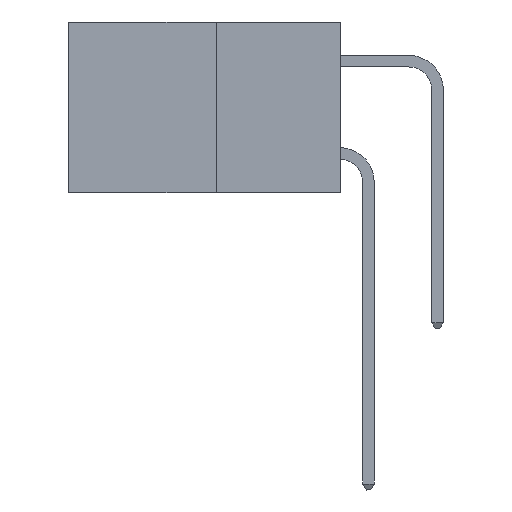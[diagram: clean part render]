
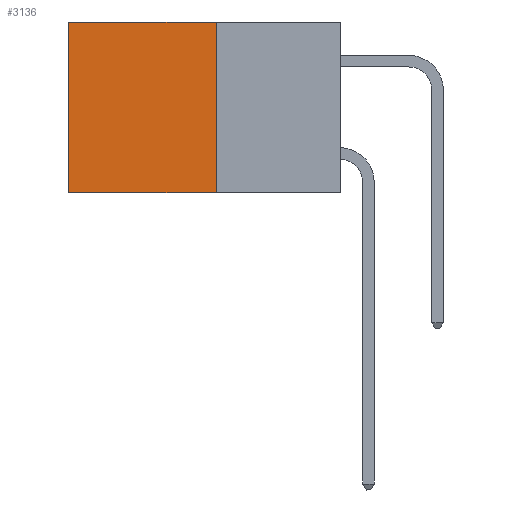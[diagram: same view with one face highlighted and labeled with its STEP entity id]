
A CAD part, left-side view. The second image highlights one B-rep face of the part: STEP entity #3136.
In plain terms, the highlighted planar face has unit normal (-1, 0, 0).
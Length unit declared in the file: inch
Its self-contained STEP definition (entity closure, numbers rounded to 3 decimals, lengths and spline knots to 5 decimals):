
#578 = LINE ( 'NONE', #8632, #11814 ) ;
#2811 = ORIENTED_EDGE ( 'NONE', *, *, #6067, .T. ) ;
#2871 = EDGE_CURVE ( 'NONE', #19294, #12877, #27606, .T. ) ;
#3136 = ADVANCED_FACE ( 'NONE', ( #26526 ), #15058, .F. ) ;
#6067 = EDGE_CURVE ( 'NONE', #19294, #20197, #23130, .T. ) ;
#6079 = CARTESIAN_POINT ( 'NONE',  ( 0.277, 0.59, -0.37 ) ) ;
#8632 = CARTESIAN_POINT ( 'NONE',  ( 0.277, 0.59, -0.37 ) ) ;
#8662 = CARTESIAN_POINT ( 'NONE',  ( 0.277, 0.27, -0.37 ) ) ;
#9228 = ORIENTED_EDGE ( 'NONE', *, *, #24205, .T. ) ;
#10613 = VECTOR ( 'NONE', #25537, 39.37008 ) ;
#10832 = CARTESIAN_POINT ( 'NONE',  ( 0.277, 0.27, 0. ) ) ;
#10877 = DIRECTION ( 'NONE',  ( 0., 0., -1. ) ) ;
#11814 = VECTOR ( 'NONE', #10877, 39.37008 ) ;
#12596 = ORIENTED_EDGE ( 'NONE', *, *, #24712, .F. ) ;
#12877 = VERTEX_POINT ( 'NONE', #8662 ) ;
#14451 = CARTESIAN_POINT ( 'NONE',  ( 0.277, 0.27, 0. ) ) ;
#14726 = DIRECTION ( 'NONE',  ( 0., 0., -1. ) ) ;
#14819 = DIRECTION ( 'NONE',  ( 1., 0., 0. ) ) ;
#15058 = PLANE ( 'NONE',  #26820 ) ;
#15574 = CARTESIAN_POINT ( 'NONE',  ( 0.277, 0.27, -0.37 ) ) ;
#16291 = VECTOR ( 'NONE', #23583, 39.37008 ) ;
#16881 = ORIENTED_EDGE ( 'NONE', *, *, #2871, .F. ) ;
#17497 = CARTESIAN_POINT ( 'NONE',  ( 0.277, 0.59, 0. ) ) ;
#17506 = DIRECTION ( 'NONE',  ( 0., 1., 0. ) ) ;
#17932 = EDGE_LOOP ( 'NONE', ( #9228, #12596, #16881, #2811 ) ) ;
#19294 = VERTEX_POINT ( 'NONE', #14451 ) ;
#20197 = VERTEX_POINT ( 'NONE', #17497 ) ;
#21374 = CARTESIAN_POINT ( 'NONE',  ( 0.277, 0.27, -0.37 ) ) ;
#22228 = LINE ( 'NONE', #21374, #16291 ) ;
#23130 = LINE ( 'NONE', #10832, #28332 ) ;
#23583 = DIRECTION ( 'NONE',  ( 0., 1., 0. ) ) ;
#24205 = EDGE_CURVE ( 'NONE', #20197, #24796, #578, .T. ) ;
#24712 = EDGE_CURVE ( 'NONE', #12877, #24796, #22228, .T. ) ;
#24796 = VERTEX_POINT ( 'NONE', #6079 ) ;
#25504 = CARTESIAN_POINT ( 'NONE',  ( 0.277, 0.27, -0.37 ) ) ;
#25537 = DIRECTION ( 'NONE',  ( 0., 0., -1. ) ) ;
#26526 = FACE_OUTER_BOUND ( 'NONE', #17932, .T. ) ;
#26820 = AXIS2_PLACEMENT_3D ( 'NONE', #15574, #14819, #14726 ) ;
#27606 = LINE ( 'NONE', #25504, #10613 ) ;
#28332 = VECTOR ( 'NONE', #17506, 39.37008 ) ;
